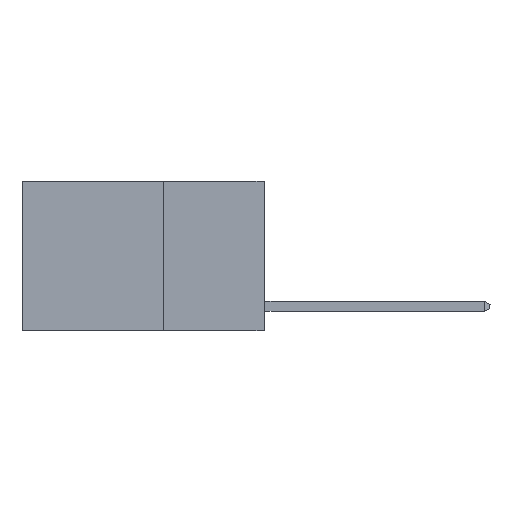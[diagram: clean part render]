
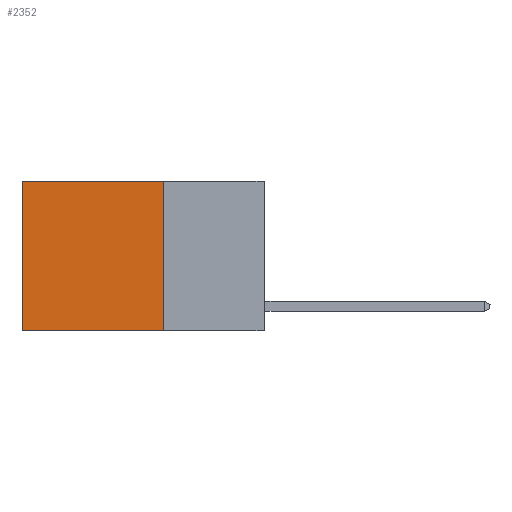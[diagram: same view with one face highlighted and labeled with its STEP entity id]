
A CAD part, left-side view. The second image highlights one B-rep face of the part: STEP entity #2352.
In plain terms, the highlighted planar face has unit normal (-1, 0, 0).
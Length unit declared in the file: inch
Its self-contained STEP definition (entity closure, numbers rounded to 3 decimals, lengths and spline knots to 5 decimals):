
#128 = ORIENTED_EDGE ( 'NONE', *, *, #771, .T. ) ;
#368 = CARTESIAN_POINT ( 'NONE',  ( 0.2625, 0.25, -0.37 ) ) ;
#457 = DIRECTION ( 'NONE',  ( 0., 1., 0. ) ) ;
#579 = CARTESIAN_POINT ( 'NONE',  ( 0.2625, 0.25, 0. ) ) ;
#614 = EDGE_LOOP ( 'NONE', ( #7899, #5844, #2182, #128 ) ) ;
#771 = EDGE_CURVE ( 'NONE', #2831, #1204, #1499, .T. ) ;
#1204 = VERTEX_POINT ( 'NONE', #5085 ) ;
#1492 = CARTESIAN_POINT ( 'NONE',  ( 0.2625, 0.25, 0. ) ) ;
#1499 = LINE ( 'NONE', #10023, #3815 ) ;
#1776 = CARTESIAN_POINT ( 'NONE',  ( 0.2625, 0.25, 0. ) ) ;
#2027 = DIRECTION ( 'NONE',  ( 0., 0., -1. ) ) ;
#2182 = ORIENTED_EDGE ( 'NONE', *, *, #8630, .F. ) ;
#2352 = ADVANCED_FACE ( 'NONE', ( #3322 ), #5414, .F. ) ;
#2596 = DIRECTION ( 'NONE',  ( 0., 0., -1. ) ) ;
#2831 = VERTEX_POINT ( 'NONE', #1492 ) ;
#2847 = AXIS2_PLACEMENT_3D ( 'NONE', #579, #5808, #2596 ) ;
#3060 = VECTOR ( 'NONE', #5812, 39.37008 ) ;
#3181 = CARTESIAN_POINT ( 'NONE',  ( 0.2625, 0.6, -0.37 ) ) ;
#3322 = FACE_OUTER_BOUND ( 'NONE', #614, .T. ) ;
#3589 = CARTESIAN_POINT ( 'NONE',  ( 0.2625, 0.6, 0. ) ) ;
#3815 = VECTOR ( 'NONE', #457, 39.37008 ) ;
#4066 = EDGE_CURVE ( 'NONE', #9721, #7264, #4873, .T. ) ;
#4873 = LINE ( 'NONE', #368, #3060 ) ;
#5085 = CARTESIAN_POINT ( 'NONE',  ( 0.2625, 0.6, 0. ) ) ;
#5414 = PLANE ( 'NONE',  #2847 ) ;
#5808 = DIRECTION ( 'NONE',  ( 1., 0., 0. ) ) ;
#5812 = DIRECTION ( 'NONE',  ( 0., 1., 0. ) ) ;
#5844 = ORIENTED_EDGE ( 'NONE', *, *, #4066, .F. ) ;
#5963 = LINE ( 'NONE', #3589, #8242 ) ;
#6029 = EDGE_CURVE ( 'NONE', #1204, #7264, #5963, .T. ) ;
#6280 = LINE ( 'NONE', #1776, #8312 ) ;
#6998 = CARTESIAN_POINT ( 'NONE',  ( 0.2625, 0.25, -0.37 ) ) ;
#7264 = VERTEX_POINT ( 'NONE', #3181 ) ;
#7899 = ORIENTED_EDGE ( 'NONE', *, *, #6029, .T. ) ;
#7981 = DIRECTION ( 'NONE',  ( 0., 0., -1. ) ) ;
#8242 = VECTOR ( 'NONE', #2027, 39.37008 ) ;
#8312 = VECTOR ( 'NONE', #7981, 39.37008 ) ;
#8630 = EDGE_CURVE ( 'NONE', #2831, #9721, #6280, .T. ) ;
#9721 = VERTEX_POINT ( 'NONE', #6998 ) ;
#10023 = CARTESIAN_POINT ( 'NONE',  ( 0.2625, 0.25, 0. ) ) ;
